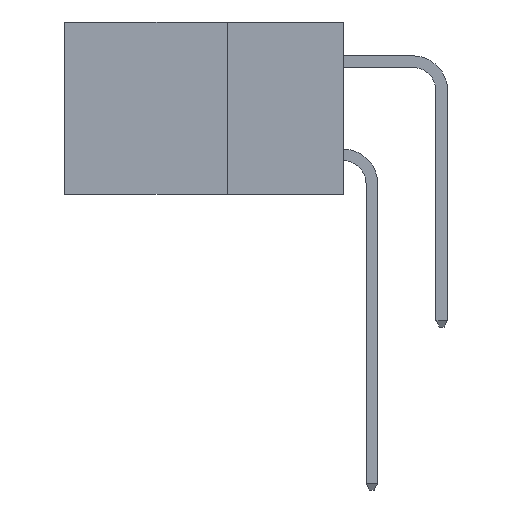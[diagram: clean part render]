
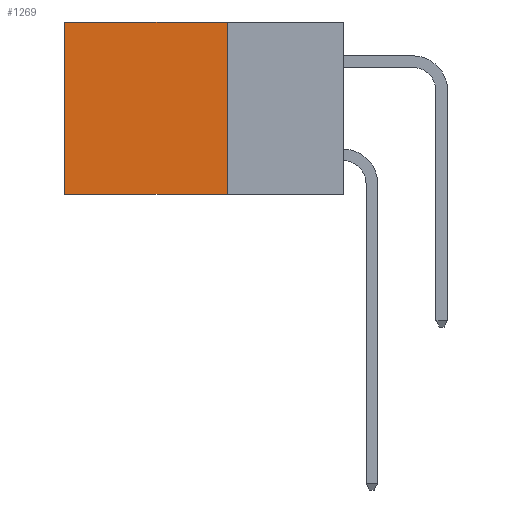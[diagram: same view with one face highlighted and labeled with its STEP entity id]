
A CAD part, left-side view. The second image highlights one B-rep face of the part: STEP entity #1269.
In plain terms, the highlighted planar face has unit normal (-1, 0, 0).
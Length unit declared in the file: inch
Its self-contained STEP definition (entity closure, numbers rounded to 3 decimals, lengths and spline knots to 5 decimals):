
#1269 = ADVANCED_FACE ( 'NONE', ( #16627 ), #3140, .F. ) ;
#1523 = CARTESIAN_POINT ( 'NONE',  ( 0.2615, 0.25, -0.37 ) ) ;
#1601 = ORIENTED_EDGE ( 'NONE', *, *, #18757, .T. ) ;
#1872 = EDGE_CURVE ( 'NONE', #20672, #15148, #13468, .T. ) ;
#1924 = VECTOR ( 'NONE', #3087, 39.37008 ) ;
#1990 = CARTESIAN_POINT ( 'NONE',  ( 0.2615, 0.25, -0.37 ) ) ;
#3087 = DIRECTION ( 'NONE',  ( 0., 1., 0. ) ) ;
#3140 = PLANE ( 'NONE',  #13852 ) ;
#5289 = DIRECTION ( 'NONE',  ( 0., 0., -1. ) ) ;
#5292 = DIRECTION ( 'NONE',  ( 1., 0., 0. ) ) ;
#6369 = ORIENTED_EDGE ( 'NONE', *, *, #1872, .T. ) ;
#6491 = LINE ( 'NONE', #7481, #7063 ) ;
#6608 = CARTESIAN_POINT ( 'NONE',  ( 0.2615, 0.25, 0. ) ) ;
#7063 = VECTOR ( 'NONE', #12652, 39.37008 ) ;
#7481 = CARTESIAN_POINT ( 'NONE',  ( 0.2615, 0.25, -0.37 ) ) ;
#8074 = ORIENTED_EDGE ( 'NONE', *, *, #16572, .F. ) ;
#10350 = DIRECTION ( 'NONE',  ( 0., 0., -1. ) ) ;
#11183 = EDGE_CURVE ( 'NONE', #19904, #14225, #14463, .T. ) ;
#11254 = LINE ( 'NONE', #6608, #1924 ) ;
#12652 = DIRECTION ( 'NONE',  ( 0., 1., 0. ) ) ;
#13468 = LINE ( 'NONE', #20820, #17419 ) ;
#13852 = AXIS2_PLACEMENT_3D ( 'NONE', #1990, #5292, #5289 ) ;
#14225 = VERTEX_POINT ( 'NONE', #17254 ) ;
#14463 = LINE ( 'NONE', #1523, #18884 ) ;
#14799 = CARTESIAN_POINT ( 'NONE',  ( 0.2615, 0.6, -0.37 ) ) ;
#15074 = CARTESIAN_POINT ( 'NONE',  ( 0.2615, 0.6, 0. ) ) ;
#15148 = VERTEX_POINT ( 'NONE', #14799 ) ;
#16331 = ORIENTED_EDGE ( 'NONE', *, *, #11183, .F. ) ;
#16572 = EDGE_CURVE ( 'NONE', #14225, #15148, #6491, .T. ) ;
#16627 = FACE_OUTER_BOUND ( 'NONE', #19402, .T. ) ;
#17254 = CARTESIAN_POINT ( 'NONE',  ( 0.2615, 0.25, -0.37 ) ) ;
#17419 = VECTOR ( 'NONE', #17833, 39.37008 ) ;
#17833 = DIRECTION ( 'NONE',  ( 0., 0., -1. ) ) ;
#18757 = EDGE_CURVE ( 'NONE', #19904, #20672, #11254, .T. ) ;
#18884 = VECTOR ( 'NONE', #10350, 39.37008 ) ;
#19402 = EDGE_LOOP ( 'NONE', ( #6369, #8074, #16331, #1601 ) ) ;
#19904 = VERTEX_POINT ( 'NONE', #21483 ) ;
#20672 = VERTEX_POINT ( 'NONE', #15074 ) ;
#20820 = CARTESIAN_POINT ( 'NONE',  ( 0.2615, 0.6, -0.37 ) ) ;
#21483 = CARTESIAN_POINT ( 'NONE',  ( 0.2615, 0.25, 0. ) ) ;
